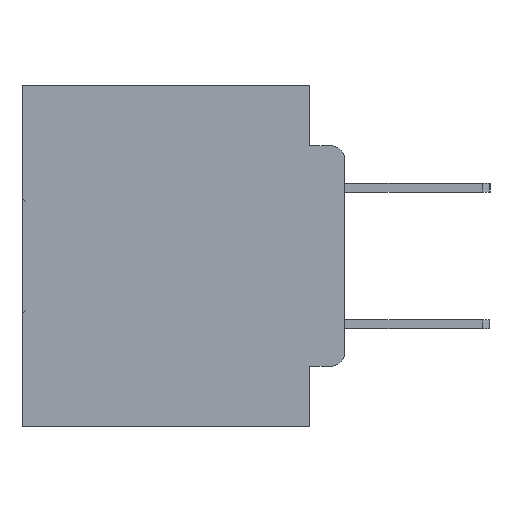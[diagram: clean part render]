
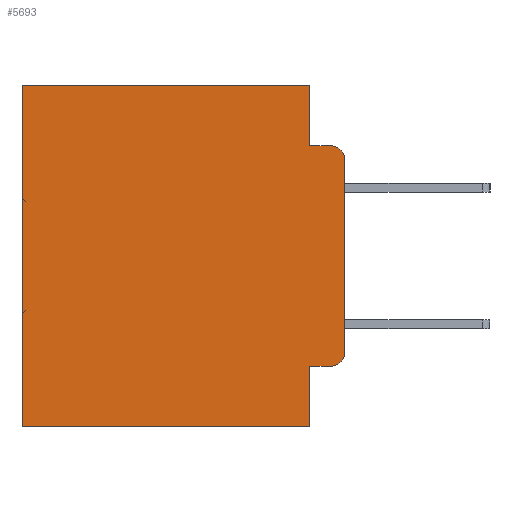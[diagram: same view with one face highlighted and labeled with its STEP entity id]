
A CAD part, left-side view. The second image highlights one B-rep face of the part: STEP entity #5693.
In plain terms, the highlighted planar face has unit normal (-1, 0, 0).
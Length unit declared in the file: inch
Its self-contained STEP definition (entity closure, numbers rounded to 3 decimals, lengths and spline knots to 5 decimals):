
#271 = VECTOR ( 'NONE', #24639, 39.37008 ) ;
#859 = CARTESIAN_POINT ( 'NONE',  ( 0.298, 0.051, 0. ) ) ;
#1214 = FACE_OUTER_BOUND ( 'NONE', #26626, .T. ) ;
#2185 = VERTEX_POINT ( 'NONE', #6495 ) ;
#2327 = DIRECTION ( 'NONE',  ( 0., 0., -1. ) ) ;
#3567 = EDGE_CURVE ( 'NONE', #4948, #20421, #7734, .T. ) ;
#3624 = CARTESIAN_POINT ( 'NONE',  ( 0.298, 0.02, -0.3915 ) ) ;
#4642 = LINE ( 'NONE', #12040, #9276 ) ;
#4948 = VERTEX_POINT ( 'NONE', #15944 ) ;
#4978 = AXIS2_PLACEMENT_3D ( 'NONE', #3624, #22366, #6358 ) ;
#5389 = EDGE_CURVE ( 'NONE', #31066, #17260, #23070, .T. ) ;
#5555 = DIRECTION ( 'NONE',  ( 0., -1., 0. ) ) ;
#5664 = CARTESIAN_POINT ( 'NONE',  ( 0.298, 0.02, -0.0885 ) ) ;
#5693 = ADVANCED_FACE ( 'NONE', ( #1214 ), #9508, .F. ) ;
#6358 = DIRECTION ( 'NONE',  ( 0., 0., -1. ) ) ;
#6495 = CARTESIAN_POINT ( 'NONE',  ( 0.298, 0.473, -0.5 ) ) ;
#7042 = CARTESIAN_POINT ( 'NONE',  ( 0.298, 0., -0.1085 ) ) ;
#7324 = LINE ( 'NONE', #26891, #27671 ) ;
#7560 = LINE ( 'NONE', #16664, #271 ) ;
#7734 = LINE ( 'NONE', #26973, #28902 ) ;
#8821 = CARTESIAN_POINT ( 'NONE',  ( 0.298, 0., -0.3915 ) ) ;
#8880 = LINE ( 'NONE', #34025, #22232 ) ;
#9276 = VECTOR ( 'NONE', #25328, 39.37008 ) ;
#9508 = PLANE ( 'NONE',  #25309 ) ;
#9564 = VECTOR ( 'NONE', #12473, 39.37008 ) ;
#9693 = DIRECTION ( 'NONE',  ( 0., 0., -1. ) ) ;
#9767 = DIRECTION ( 'NONE',  ( 1., 0., 0. ) ) ;
#10211 = DIRECTION ( 'NONE',  ( -1., 0., 0. ) ) ;
#11061 = LINE ( 'NONE', #19546, #24390 ) ;
#11896 = EDGE_CURVE ( 'NONE', #12736, #22054, #7560, .T. ) ;
#12040 = CARTESIAN_POINT ( 'NONE',  ( 0.298, 0.051, -0.4115 ) ) ;
#12473 = DIRECTION ( 'NONE',  ( 0., 1., 0. ) ) ;
#12551 = CARTESIAN_POINT ( 'NONE',  ( 0.298, 0., 0. ) ) ;
#12703 = CARTESIAN_POINT ( 'NONE',  ( 0.298, 0.051, -0.0885 ) ) ;
#12736 = VERTEX_POINT ( 'NONE', #7042 ) ;
#12783 = ORIENTED_EDGE ( 'NONE', *, *, #11896, .F. ) ;
#13922 = ORIENTED_EDGE ( 'NONE', *, *, #17957, .F. ) ;
#14789 = AXIS2_PLACEMENT_3D ( 'NONE', #26162, #10211, #28760 ) ;
#15755 = EDGE_CURVE ( 'NONE', #20421, #2185, #23717, .T. ) ;
#15944 = CARTESIAN_POINT ( 'NONE',  ( 0.298, 0.051, -0.4115 ) ) ;
#16015 = VECTOR ( 'NONE', #5555, 39.37008 ) ;
#16664 = CARTESIAN_POINT ( 'NONE',  ( 0.298, 0., 0. ) ) ;
#17260 = VERTEX_POINT ( 'NONE', #5664 ) ;
#17957 = EDGE_CURVE ( 'NONE', #19291, #31066, #11061, .T. ) ;
#18598 = ORIENTED_EDGE ( 'NONE', *, *, #33680, .T. ) ;
#19110 = ORIENTED_EDGE ( 'NONE', *, *, #27478, .T. ) ;
#19150 = ORIENTED_EDGE ( 'NONE', *, *, #3567, .F. ) ;
#19192 = CARTESIAN_POINT ( 'NONE',  ( 0.298, 0.051, -0.0885 ) ) ;
#19291 = VERTEX_POINT ( 'NONE', #859 ) ;
#19546 = CARTESIAN_POINT ( 'NONE',  ( 0.298, 0.051, 0. ) ) ;
#19654 = CARTESIAN_POINT ( 'NONE',  ( 0.298, 0.473, 0. ) ) ;
#20417 = EDGE_CURVE ( 'NONE', #4948, #24027, #4642, .T. ) ;
#20421 = VERTEX_POINT ( 'NONE', #28076 ) ;
#20438 = CARTESIAN_POINT ( 'NONE',  ( 0.298, 0., -0.5 ) ) ;
#22054 = VERTEX_POINT ( 'NONE', #8821 ) ;
#22232 = VECTOR ( 'NONE', #2327, 39.37008 ) ;
#22366 = DIRECTION ( 'NONE',  ( -1., 0., 0. ) ) ;
#23070 = LINE ( 'NONE', #19192, #16015 ) ;
#23717 = LINE ( 'NONE', #20438, #9564 ) ;
#24027 = VERTEX_POINT ( 'NONE', #33412 ) ;
#24390 = VECTOR ( 'NONE', #27509, 39.37008 ) ;
#24639 = DIRECTION ( 'NONE',  ( 0., 0., -1. ) ) ;
#24858 = EDGE_CURVE ( 'NONE', #19291, #30224, #7324, .T. ) ;
#25309 = AXIS2_PLACEMENT_3D ( 'NONE', #12551, #9767, #9693 ) ;
#25328 = DIRECTION ( 'NONE',  ( 0., -1., 0. ) ) ;
#26162 = CARTESIAN_POINT ( 'NONE',  ( 0.298, 0.02, -0.1085 ) ) ;
#26626 = EDGE_LOOP ( 'NONE', ( #12783, #18598, #28941, #13922, #28552, #30769, #28186, #19150, #30082, #19110 ) ) ;
#26891 = CARTESIAN_POINT ( 'NONE',  ( 0.298, 0., 0. ) ) ;
#26973 = CARTESIAN_POINT ( 'NONE',  ( 0.298, 0.051, 0. ) ) ;
#27244 = CIRCLE ( 'NONE', #14789, 0.02 ) ;
#27342 = DIRECTION ( 'NONE',  ( 0., 0., -1. ) ) ;
#27478 = EDGE_CURVE ( 'NONE', #24027, #22054, #30390, .T. ) ;
#27509 = DIRECTION ( 'NONE',  ( 0., 0., -1. ) ) ;
#27671 = VECTOR ( 'NONE', #29513, 39.37008 ) ;
#28076 = CARTESIAN_POINT ( 'NONE',  ( 0.298, 0.051, -0.5 ) ) ;
#28186 = ORIENTED_EDGE ( 'NONE', *, *, #15755, .F. ) ;
#28552 = ORIENTED_EDGE ( 'NONE', *, *, #24858, .T. ) ;
#28760 = DIRECTION ( 'NONE',  ( 0., 0., -1. ) ) ;
#28902 = VECTOR ( 'NONE', #27342, 39.37008 ) ;
#28941 = ORIENTED_EDGE ( 'NONE', *, *, #5389, .F. ) ;
#29233 = EDGE_CURVE ( 'NONE', #30224, #2185, #8880, .T. ) ;
#29513 = DIRECTION ( 'NONE',  ( 0., 1., 0. ) ) ;
#30082 = ORIENTED_EDGE ( 'NONE', *, *, #20417, .T. ) ;
#30224 = VERTEX_POINT ( 'NONE', #19654 ) ;
#30390 = CIRCLE ( 'NONE', #4978, 0.02 ) ;
#30769 = ORIENTED_EDGE ( 'NONE', *, *, #29233, .T. ) ;
#31066 = VERTEX_POINT ( 'NONE', #12703 ) ;
#33412 = CARTESIAN_POINT ( 'NONE',  ( 0.298, 0.02, -0.4115 ) ) ;
#33680 = EDGE_CURVE ( 'NONE', #12736, #17260, #27244, .T. ) ;
#34025 = CARTESIAN_POINT ( 'NONE',  ( 0.298, 0.473, 0. ) ) ;
